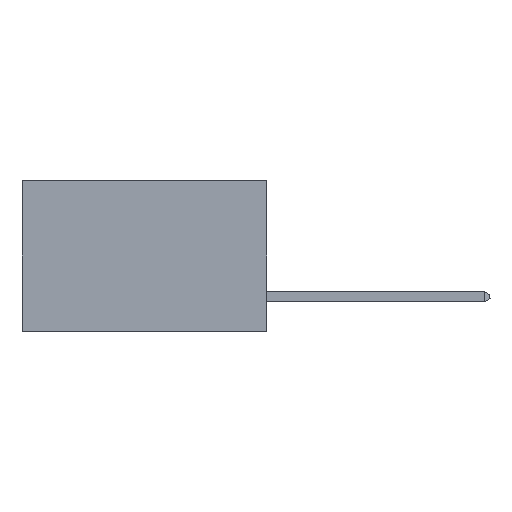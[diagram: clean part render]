
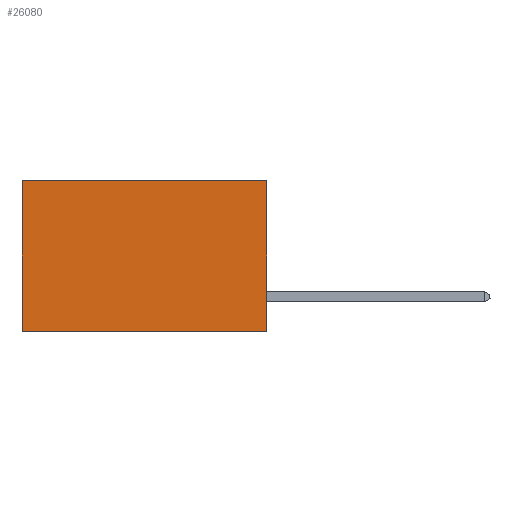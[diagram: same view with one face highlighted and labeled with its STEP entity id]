
A CAD part, left-side view. The second image highlights one B-rep face of the part: STEP entity #26080.
In plain terms, the highlighted planar face has unit normal (-1, 0, 0).
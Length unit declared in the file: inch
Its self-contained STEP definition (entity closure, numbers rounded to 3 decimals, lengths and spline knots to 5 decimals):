
#2819 = CARTESIAN_POINT ( 'NONE',  ( 0.2875, 0.6, -0.37 ) ) ;
#2956 = LINE ( 'NONE', #6567, #7910 ) ;
#3377 = VECTOR ( 'NONE', #28788, 39.37008 ) ;
#3662 = LINE ( 'NONE', #12549, #4637 ) ;
#4637 = VECTOR ( 'NONE', #24144, 39.37008 ) ;
#5663 = VERTEX_POINT ( 'NONE', #8691 ) ;
#6567 = CARTESIAN_POINT ( 'NONE',  ( 0.2875, 0.6, 0. ) ) ;
#6659 = ORIENTED_EDGE ( 'NONE', *, *, #17942, .T. ) ;
#7910 = VECTOR ( 'NONE', #25491, 39.37008 ) ;
#8691 = CARTESIAN_POINT ( 'NONE',  ( 0.2875, 0., -0.37 ) ) ;
#8827 = VECTOR ( 'NONE', #23077, 39.37008 ) ;
#8875 = CARTESIAN_POINT ( 'NONE',  ( 0.2875, 0., 0. ) ) ;
#12093 = LINE ( 'NONE', #25290, #8827 ) ;
#12549 = CARTESIAN_POINT ( 'NONE',  ( 0.2875, 0., -0.37 ) ) ;
#13381 = EDGE_CURVE ( 'NONE', #23223, #22240, #12093, .T. ) ;
#14740 = ORIENTED_EDGE ( 'NONE', *, *, #17486, .F. ) ;
#16048 = EDGE_CURVE ( 'NONE', #5663, #29949, #3662, .T. ) ;
#17486 = EDGE_CURVE ( 'NONE', #23223, #5663, #33385, .T. ) ;
#17942 = EDGE_CURVE ( 'NONE', #22240, #29949, #2956, .T. ) ;
#20681 = FACE_OUTER_BOUND ( 'NONE', #30076, .T. ) ;
#22240 = VERTEX_POINT ( 'NONE', #25622 ) ;
#23077 = DIRECTION ( 'NONE',  ( 0., 1., 0. ) ) ;
#23223 = VERTEX_POINT ( 'NONE', #30540 ) ;
#24144 = DIRECTION ( 'NONE',  ( 0., 1., 0. ) ) ;
#25290 = CARTESIAN_POINT ( 'NONE',  ( 0.2875, 0., 0. ) ) ;
#25491 = DIRECTION ( 'NONE',  ( 0., 0., -1. ) ) ;
#25622 = CARTESIAN_POINT ( 'NONE',  ( 0.2875, 0.6, 0. ) ) ;
#26080 = ADVANCED_FACE ( 'NONE', ( #20681 ), #36221, .F. ) ;
#28061 = CARTESIAN_POINT ( 'NONE',  ( 0.2875, 0., 0. ) ) ;
#28788 = DIRECTION ( 'NONE',  ( 0., 0., -1. ) ) ;
#29949 = VERTEX_POINT ( 'NONE', #2819 ) ;
#30044 = AXIS2_PLACEMENT_3D ( 'NONE', #28061, #34195, #34302 ) ;
#30076 = EDGE_LOOP ( 'NONE', ( #6659, #31194, #14740, #32835 ) ) ;
#30540 = CARTESIAN_POINT ( 'NONE',  ( 0.2875, 0., 0. ) ) ;
#31194 = ORIENTED_EDGE ( 'NONE', *, *, #16048, .F. ) ;
#32835 = ORIENTED_EDGE ( 'NONE', *, *, #13381, .T. ) ;
#33385 = LINE ( 'NONE', #8875, #3377 ) ;
#34195 = DIRECTION ( 'NONE',  ( 1., 0., 0. ) ) ;
#34302 = DIRECTION ( 'NONE',  ( 0., 0., -1. ) ) ;
#36221 = PLANE ( 'NONE',  #30044 ) ;
